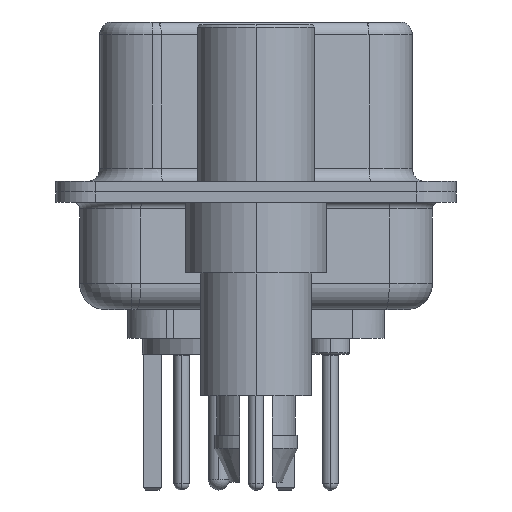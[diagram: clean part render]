
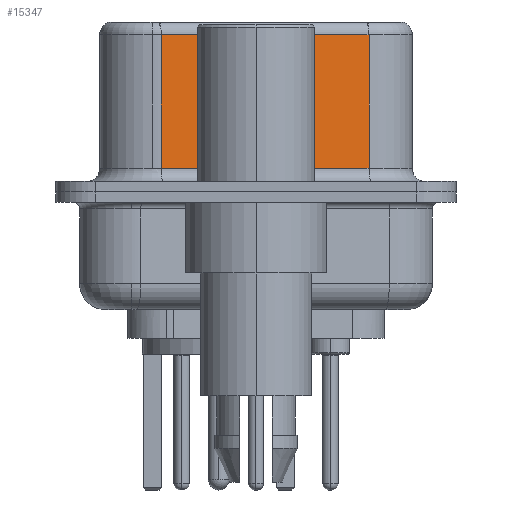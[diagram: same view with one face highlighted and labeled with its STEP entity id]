
A CAD part, left-side view. The second image highlights one B-rep face of the part: STEP entity #15347.
In plain terms, the highlighted planar face has unit normal (-0.985, -0.174, 0).
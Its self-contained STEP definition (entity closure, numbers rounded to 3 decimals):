
#1002 = ORIENTED_EDGE ( 'NONE', *, *, #7393, .T. ) ;
#1290 = CARTESIAN_POINT ( 'NONE',  ( 5.132, -4.322, 6.52 ) ) ;
#1501 = ORIENTED_EDGE ( 'NONE', *, *, #7806, .T. ) ;
#1594 = CARTESIAN_POINT ( 'NONE',  ( 5.132, -4.322, 0.9 ) ) ;
#1756 = CARTESIAN_POINT ( 'NONE',  ( 5.132, -4.322, 6.02 ) ) ;
#2273 = DIRECTION ( 'NONE',  ( 0.174, -0.985, 0. ) ) ;
#3253 = CARTESIAN_POINT ( 'NONE',  ( 5.132, -4.322, 6.02 ) ) ;
#4472 = EDGE_LOOP ( 'NONE', ( #9158, #21176, #1501, #1002 ) ) ;
#5573 = LINE ( 'NONE', #15892, #10909 ) ;
#6788 = CARTESIAN_POINT ( 'NONE',  ( 3.73, 3.628, 0.9 ) ) ;
#7393 = EDGE_CURVE ( 'NONE', #24823, #26665, #5573, .T. ) ;
#7806 = EDGE_CURVE ( 'NONE', #12550, #24823, #28381, .T. ) ;
#7884 = DIRECTION ( 'NONE',  ( -0.174, 0.985, 0. ) ) ;
#9158 = ORIENTED_EDGE ( 'NONE', *, *, #18502, .F. ) ;
#9282 = FACE_OUTER_BOUND ( 'NONE', #4472, .T. ) ;
#9336 = PLANE ( 'NONE',  #12791 ) ;
#9536 = LINE ( 'NONE', #1290, #26718 ) ;
#10909 = VECTOR ( 'NONE', #2273, 1000. ) ;
#11609 = DIRECTION ( 'NONE',  ( 0.985, 0.174, 0. ) ) ;
#12550 = VERTEX_POINT ( 'NONE', #27656 ) ;
#12791 = AXIS2_PLACEMENT_3D ( 'NONE', #25045, #11609, #27242 ) ;
#15347 = ADVANCED_FACE ( 'NONE', ( #9282 ), #9336, .F. ) ;
#15848 = VECTOR ( 'NONE', #25960, 1000. ) ;
#15892 = CARTESIAN_POINT ( 'NONE',  ( 5.132, -4.322, 0.9 ) ) ;
#18502 = EDGE_CURVE ( 'NONE', #27291, #26665, #9536, .T. ) ;
#19230 = EDGE_CURVE ( 'NONE', #27291, #12550, #23932, .T. ) ;
#19422 = DIRECTION ( 'NONE',  ( 0., 0., -1. ) ) ;
#21176 = ORIENTED_EDGE ( 'NONE', *, *, #19230, .T. ) ;
#21423 = CARTESIAN_POINT ( 'NONE',  ( 3.73, 3.628, 6.52 ) ) ;
#23216 = VECTOR ( 'NONE', #7884, 1000. ) ;
#23932 = LINE ( 'NONE', #3253, #23216 ) ;
#24823 = VERTEX_POINT ( 'NONE', #6788 ) ;
#25045 = CARTESIAN_POINT ( 'NONE',  ( 5.132, -4.322, 6.52 ) ) ;
#25960 = DIRECTION ( 'NONE',  ( 0., 0., -1. ) ) ;
#26665 = VERTEX_POINT ( 'NONE', #1594 ) ;
#26718 = VECTOR ( 'NONE', #19422, 1000. ) ;
#27242 = DIRECTION ( 'NONE',  ( -0.174, 0.985, 0. ) ) ;
#27291 = VERTEX_POINT ( 'NONE', #1756 ) ;
#27656 = CARTESIAN_POINT ( 'NONE',  ( 3.73, 3.628, 6.02 ) ) ;
#28381 = LINE ( 'NONE', #21423, #15848 ) ;
